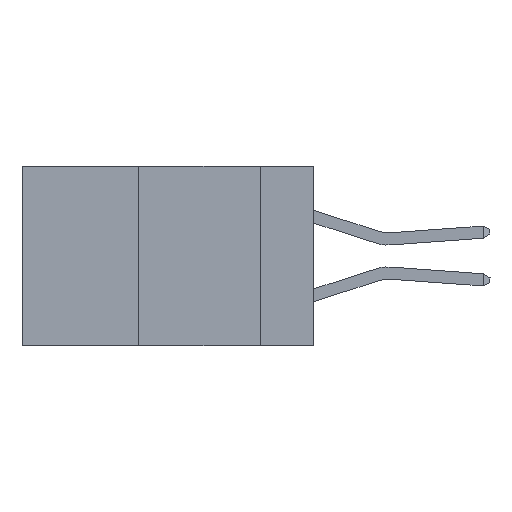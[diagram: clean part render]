
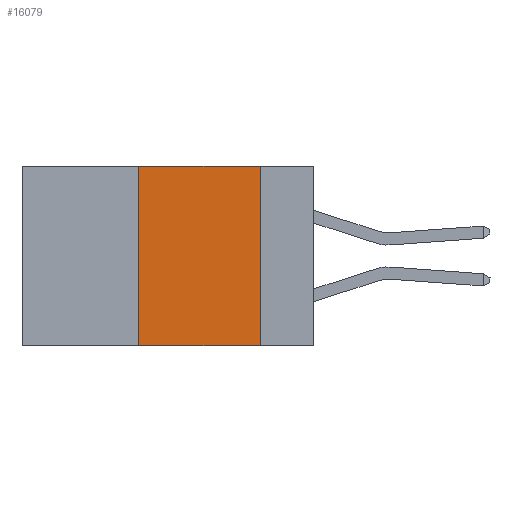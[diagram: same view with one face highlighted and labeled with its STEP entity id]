
A CAD part, left-side view. The second image highlights one B-rep face of the part: STEP entity #16079.
In plain terms, the highlighted planar face has unit normal (-1, 0, 0).
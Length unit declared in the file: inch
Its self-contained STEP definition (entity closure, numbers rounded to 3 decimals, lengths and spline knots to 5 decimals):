
#930 = DIRECTION ( 'NONE',  ( 0., 0., -1. ) ) ;
#1148 = ORIENTED_EDGE ( 'NONE', *, *, #8956, .F. ) ;
#1800 = VECTOR ( 'NONE', #7616, 39.37008 ) ;
#2850 = CARTESIAN_POINT ( 'NONE',  ( 0., 0.6, 0. ) ) ;
#3637 = VERTEX_POINT ( 'NONE', #19492 ) ;
#3736 = CARTESIAN_POINT ( 'NONE',  ( 0., 0.11, -0.37 ) ) ;
#3751 = ORIENTED_EDGE ( 'NONE', *, *, #11755, .T. ) ;
#3821 = VECTOR ( 'NONE', #17184, 39.37008 ) ;
#4020 = AXIS2_PLACEMENT_3D ( 'NONE', #2850, #4633, #16831 ) ;
#4633 = DIRECTION ( 'NONE',  ( 1., 0., 0. ) ) ;
#5904 = FACE_OUTER_BOUND ( 'NONE', #20761, .T. ) ;
#6095 = CARTESIAN_POINT ( 'NONE',  ( 0., 0.11, 0. ) ) ;
#6614 = VERTEX_POINT ( 'NONE', #8652 ) ;
#7059 = EDGE_CURVE ( 'NONE', #16993, #3637, #17136, .T. ) ;
#7616 = DIRECTION ( 'NONE',  ( 0., -1., 0. ) ) ;
#8652 = CARTESIAN_POINT ( 'NONE',  ( 0., 0.11, 0. ) ) ;
#8956 = EDGE_CURVE ( 'NONE', #3637, #6614, #15161, .T. ) ;
#9108 = LINE ( 'NONE', #18851, #3821 ) ;
#11755 = EDGE_CURVE ( 'NONE', #16993, #17539, #9108, .T. ) ;
#13367 = PLANE ( 'NONE',  #4020 ) ;
#13968 = LINE ( 'NONE', #6095, #18026 ) ;
#15161 = LINE ( 'NONE', #17993, #1800 ) ;
#16079 = ADVANCED_FACE ( 'NONE', ( #5904 ), #13367, .F. ) ;
#16831 = DIRECTION ( 'NONE',  ( 0., 0., -1. ) ) ;
#16993 = VERTEX_POINT ( 'NONE', #17475 ) ;
#17136 = LINE ( 'NONE', #18377, #17678 ) ;
#17184 = DIRECTION ( 'NONE',  ( 0., -1., 0. ) ) ;
#17475 = CARTESIAN_POINT ( 'NONE',  ( 0., 0.36, -0.37 ) ) ;
#17539 = VERTEX_POINT ( 'NONE', #3736 ) ;
#17678 = VECTOR ( 'NONE', #20115, 39.37008 ) ;
#17993 = CARTESIAN_POINT ( 'NONE',  ( 0., 0.6, 0. ) ) ;
#18026 = VECTOR ( 'NONE', #930, 39.37008 ) ;
#18377 = CARTESIAN_POINT ( 'NONE',  ( 0., 0.36, 0. ) ) ;
#18851 = CARTESIAN_POINT ( 'NONE',  ( 0., 0.6, -0.37 ) ) ;
#19000 = EDGE_CURVE ( 'NONE', #6614, #17539, #13968, .T. ) ;
#19492 = CARTESIAN_POINT ( 'NONE',  ( 0., 0.36, 0. ) ) ;
#20115 = DIRECTION ( 'NONE',  ( 0., 0., 1. ) ) ;
#20530 = ORIENTED_EDGE ( 'NONE', *, *, #19000, .F. ) ;
#20761 = EDGE_LOOP ( 'NONE', ( #20530, #1148, #22299, #3751 ) ) ;
#22299 = ORIENTED_EDGE ( 'NONE', *, *, #7059, .F. ) ;
